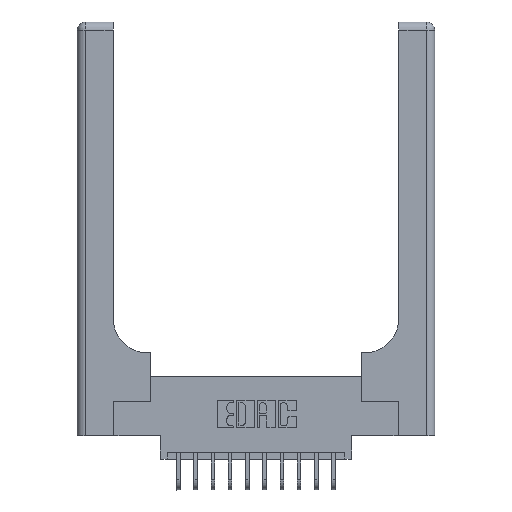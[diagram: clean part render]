
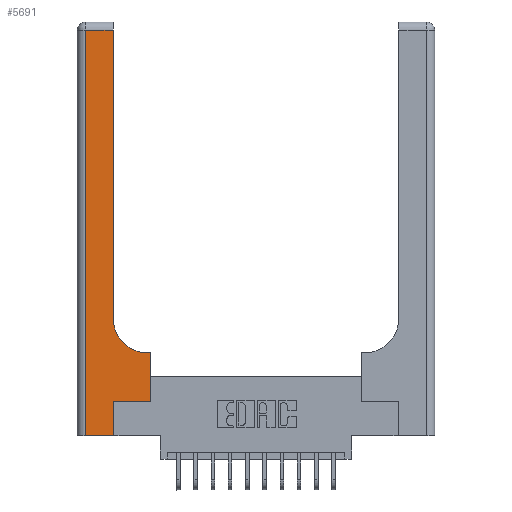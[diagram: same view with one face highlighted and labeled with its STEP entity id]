
A CAD part, top view. The second image highlights one B-rep face of the part: STEP entity #5691.
In plain terms, the highlighted planar face has unit normal (0, 0, 1).
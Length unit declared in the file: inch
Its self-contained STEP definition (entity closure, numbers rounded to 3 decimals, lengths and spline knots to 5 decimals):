
#393 = CARTESIAN_POINT ( 'NONE',  ( 0.06, 3., 0.37 ) ) ;
#429 = LINE ( 'NONE', #6324, #15996 ) ;
#877 = VERTEX_POINT ( 'NONE', #1286 ) ;
#1285 = ORIENTED_EDGE ( 'NONE', *, *, #1867, .T. ) ;
#1286 = CARTESIAN_POINT ( 'NONE',  ( 0.528, 0.6, 0.37 ) ) ;
#1333 = VERTEX_POINT ( 'NONE', #15081 ) ;
#1606 = DIRECTION ( 'NONE',  ( 0., -1., 0. ) ) ;
#1821 = ORIENTED_EDGE ( 'NONE', *, *, #8011, .T. ) ;
#1867 = EDGE_CURVE ( 'NONE', #11150, #12119, #8276, .T. ) ;
#2260 = DIRECTION ( 'NONE',  ( 0., 1., 0. ) ) ;
#3090 = PLANE ( 'NONE',  #15312 ) ;
#3343 = AXIS2_PLACEMENT_3D ( 'NONE', #9401, #9463, #17756 ) ;
#3352 = DIRECTION ( 'NONE',  ( 1., 0., 0. ) ) ;
#3742 = CARTESIAN_POINT ( 'NONE',  ( 0.26, 0.85, 0.37 ) ) ;
#3743 = ORIENTED_EDGE ( 'NONE', *, *, #5279, .T. ) ;
#3996 = VECTOR ( 'NONE', #16207, 39.37008 ) ;
#4222 = DIRECTION ( 'NONE',  ( 0., 1., 0. ) ) ;
#4752 = EDGE_CURVE ( 'NONE', #877, #9227, #8880, .T. ) ;
#5173 = VECTOR ( 'NONE', #13431, 39.37008 ) ;
#5279 = EDGE_CURVE ( 'NONE', #13716, #1333, #429, .T. ) ;
#5643 = VECTOR ( 'NONE', #2260, 39.37008 ) ;
#5691 = ADVANCED_FACE ( 'NONE', ( #9718 ), #3090, .F. ) ;
#5775 = CARTESIAN_POINT ( 'NONE',  ( 0.528, 0.25, 0.37 ) ) ;
#5949 = VERTEX_POINT ( 'NONE', #9706 ) ;
#6031 = VECTOR ( 'NONE', #3352, 39.37008 ) ;
#6309 = CARTESIAN_POINT ( 'NONE',  ( 0.265, 0.25, 0.37 ) ) ;
#6324 = CARTESIAN_POINT ( 'NONE',  ( 0., 2.94, 0.37 ) ) ;
#6372 = CARTESIAN_POINT ( 'NONE',  ( 0.265, 0., 0.37 ) ) ;
#7730 = DIRECTION ( 'NONE',  ( -1., 0., 0. ) ) ;
#7757 = CARTESIAN_POINT ( 'NONE',  ( 0.26, 2.94, 0.37 ) ) ;
#8011 = EDGE_CURVE ( 'NONE', #1333, #5949, #9879, .T. ) ;
#8142 = EDGE_CURVE ( 'NONE', #12119, #877, #14400, .T. ) ;
#8276 = LINE ( 'NONE', #6309, #12202 ) ;
#8461 = CARTESIAN_POINT ( 'NONE',  ( 0.265, 0.25, 0.37 ) ) ;
#8711 = ORIENTED_EDGE ( 'NONE', *, *, #4752, .T. ) ;
#8880 = LINE ( 'NONE', #17208, #5173 ) ;
#9124 = CARTESIAN_POINT ( 'NONE',  ( 0.51, 0.6, 0.37 ) ) ;
#9227 = VERTEX_POINT ( 'NONE', #9124 ) ;
#9401 = CARTESIAN_POINT ( 'NONE',  ( 0.51, 0.85, 0.37 ) ) ;
#9463 = DIRECTION ( 'NONE',  ( 0., 0., -1. ) ) ;
#9706 = CARTESIAN_POINT ( 'NONE',  ( 0.06, 0., 0.37 ) ) ;
#9718 = FACE_OUTER_BOUND ( 'NONE', #11629, .T. ) ;
#9879 = LINE ( 'NONE', #393, #13739 ) ;
#9922 = ORIENTED_EDGE ( 'NONE', *, *, #8142, .T. ) ;
#10424 = EDGE_CURVE ( 'NONE', #17463, #11150, #15169, .T. ) ;
#10630 = LINE ( 'NONE', #13045, #6031 ) ;
#11137 = ORIENTED_EDGE ( 'NONE', *, *, #11666, .T. ) ;
#11150 = VERTEX_POINT ( 'NONE', #8461 ) ;
#11446 = ORIENTED_EDGE ( 'NONE', *, *, #11786, .T. ) ;
#11629 = EDGE_LOOP ( 'NONE', ( #11446, #3743, #1821, #16651, #13820, #1285, #9922, #8711, #11137 ) ) ;
#11666 = EDGE_CURVE ( 'NONE', #9227, #14291, #14934, .T. ) ;
#11786 = EDGE_CURVE ( 'NONE', #14291, #13716, #15344, .T. ) ;
#12119 = VERTEX_POINT ( 'NONE', #5775 ) ;
#12202 = VECTOR ( 'NONE', #16491, 39.37008 ) ;
#12612 = DIRECTION ( 'NONE',  ( -1., 0., 0. ) ) ;
#13045 = CARTESIAN_POINT ( 'NONE',  ( 0., 0., 0.37 ) ) ;
#13431 = DIRECTION ( 'NONE',  ( -1., 0., 0. ) ) ;
#13716 = VERTEX_POINT ( 'NONE', #7757 ) ;
#13739 = VECTOR ( 'NONE', #1606, 39.37008 ) ;
#13820 = ORIENTED_EDGE ( 'NONE', *, *, #10424, .T. ) ;
#14036 = CARTESIAN_POINT ( 'NONE',  ( 0.26, 3., 0.37 ) ) ;
#14165 = DIRECTION ( 'NONE',  ( 0., 0., -1. ) ) ;
#14291 = VERTEX_POINT ( 'NONE', #3742 ) ;
#14400 = LINE ( 'NONE', #14823, #3996 ) ;
#14720 = VECTOR ( 'NONE', #4222, 39.37008 ) ;
#14823 = CARTESIAN_POINT ( 'NONE',  ( 0.528, 0.25, 0.37 ) ) ;
#14934 = CIRCLE ( 'NONE', #3343, 0.25 ) ;
#15081 = CARTESIAN_POINT ( 'NONE',  ( 0.06, 2.94, 0.37 ) ) ;
#15169 = LINE ( 'NONE', #6372, #5643 ) ;
#15312 = AXIS2_PLACEMENT_3D ( 'NONE', #16782, #14165, #12612 ) ;
#15344 = LINE ( 'NONE', #14036, #14720 ) ;
#15996 = VECTOR ( 'NONE', #7730, 39.37008 ) ;
#16207 = DIRECTION ( 'NONE',  ( 0., 1., 0. ) ) ;
#16480 = CARTESIAN_POINT ( 'NONE',  ( 0.265, 0., 0.37 ) ) ;
#16491 = DIRECTION ( 'NONE',  ( 1., 0., 0. ) ) ;
#16651 = ORIENTED_EDGE ( 'NONE', *, *, #17231, .T. ) ;
#16782 = CARTESIAN_POINT ( 'NONE',  ( 0., 3., 0.37 ) ) ;
#17208 = CARTESIAN_POINT ( 'NONE',  ( 0.26, 0.6, 0.37 ) ) ;
#17231 = EDGE_CURVE ( 'NONE', #5949, #17463, #10630, .T. ) ;
#17463 = VERTEX_POINT ( 'NONE', #16480 ) ;
#17756 = DIRECTION ( 'NONE',  ( 1., 0., 0. ) ) ;
